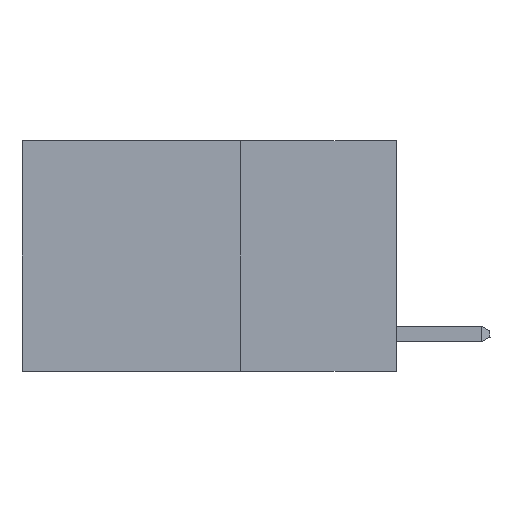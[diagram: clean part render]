
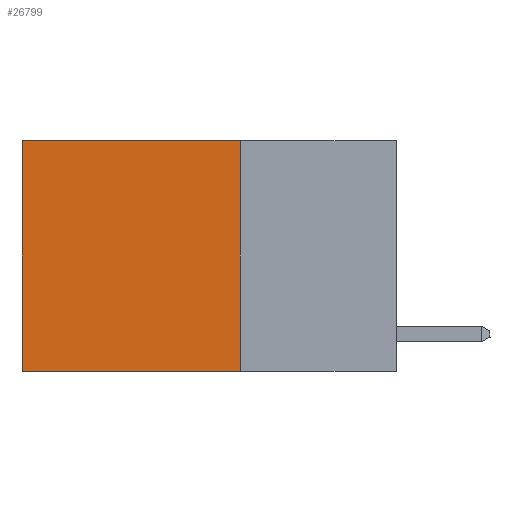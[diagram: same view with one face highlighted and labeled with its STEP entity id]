
A CAD part, left-side view. The second image highlights one B-rep face of the part: STEP entity #26799.
In plain terms, the highlighted planar face has unit normal (-1, 0, 0).
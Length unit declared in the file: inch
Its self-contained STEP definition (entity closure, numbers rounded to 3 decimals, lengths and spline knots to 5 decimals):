
#135 = DIRECTION ( 'NONE',  ( 0., 0., -1. ) ) ;
#1109 = ORIENTED_EDGE ( 'NONE', *, *, #17012, .T. ) ;
#1228 = ORIENTED_EDGE ( 'NONE', *, *, #14268, .T. ) ;
#1651 = LINE ( 'NONE', #8423, #22564 ) ;
#2195 = DIRECTION ( 'NONE',  ( 0., 1., 0. ) ) ;
#2835 = CARTESIAN_POINT ( 'NONE',  ( 0.2625, 0.25, 0. ) ) ;
#5400 = CARTESIAN_POINT ( 'NONE',  ( 0.2625, 0.25, -0.37 ) ) ;
#5627 = CARTESIAN_POINT ( 'NONE',  ( 0.2625, 0.25, 0. ) ) ;
#8423 = CARTESIAN_POINT ( 'NONE',  ( 0.2625, 0.25, 0. ) ) ;
#8612 = LINE ( 'NONE', #25177, #24602 ) ;
#8834 = ORIENTED_EDGE ( 'NONE', *, *, #20939, .F. ) ;
#8840 = VERTEX_POINT ( 'NONE', #18829 ) ;
#8911 = DIRECTION ( 'NONE',  ( 1., 0., 0. ) ) ;
#9842 = VERTEX_POINT ( 'NONE', #12313 ) ;
#11584 = VERTEX_POINT ( 'NONE', #26209 ) ;
#12313 = CARTESIAN_POINT ( 'NONE',  ( 0.2625, 0.6, -0.37 ) ) ;
#12494 = EDGE_LOOP ( 'NONE', ( #1109, #24855, #8834, #1228 ) ) ;
#12666 = VECTOR ( 'NONE', #16024, 39.37008 ) ;
#13352 = VERTEX_POINT ( 'NONE', #2835 ) ;
#14268 = EDGE_CURVE ( 'NONE', #13352, #11584, #1651, .T. ) ;
#15116 = PLANE ( 'NONE',  #20164 ) ;
#16024 = DIRECTION ( 'NONE',  ( 0., 0., -1. ) ) ;
#17012 = EDGE_CURVE ( 'NONE', #11584, #9842, #8612, .T. ) ;
#18829 = CARTESIAN_POINT ( 'NONE',  ( 0.2625, 0.25, -0.37 ) ) ;
#18929 = LINE ( 'NONE', #5400, #23827 ) ;
#19445 = EDGE_CURVE ( 'NONE', #8840, #9842, #18929, .T. ) ;
#20164 = AXIS2_PLACEMENT_3D ( 'NONE', #21403, #8911, #23481 ) ;
#20939 = EDGE_CURVE ( 'NONE', #13352, #8840, #23744, .T. ) ;
#21403 = CARTESIAN_POINT ( 'NONE',  ( 0.2625, 0.25, 0. ) ) ;
#22094 = DIRECTION ( 'NONE',  ( 0., 1., 0. ) ) ;
#22564 = VECTOR ( 'NONE', #2195, 39.37008 ) ;
#23481 = DIRECTION ( 'NONE',  ( 0., 0., -1. ) ) ;
#23744 = LINE ( 'NONE', #5627, #12666 ) ;
#23827 = VECTOR ( 'NONE', #22094, 39.37008 ) ;
#24602 = VECTOR ( 'NONE', #135, 39.37008 ) ;
#24855 = ORIENTED_EDGE ( 'NONE', *, *, #19445, .F. ) ;
#25050 = FACE_OUTER_BOUND ( 'NONE', #12494, .T. ) ;
#25177 = CARTESIAN_POINT ( 'NONE',  ( 0.2625, 0.6, 0. ) ) ;
#26209 = CARTESIAN_POINT ( 'NONE',  ( 0.2625, 0.6, 0. ) ) ;
#26799 = ADVANCED_FACE ( 'NONE', ( #25050 ), #15116, .F. ) ;
